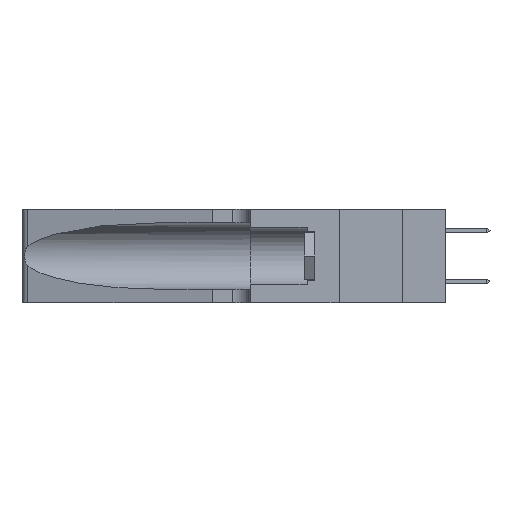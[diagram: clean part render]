
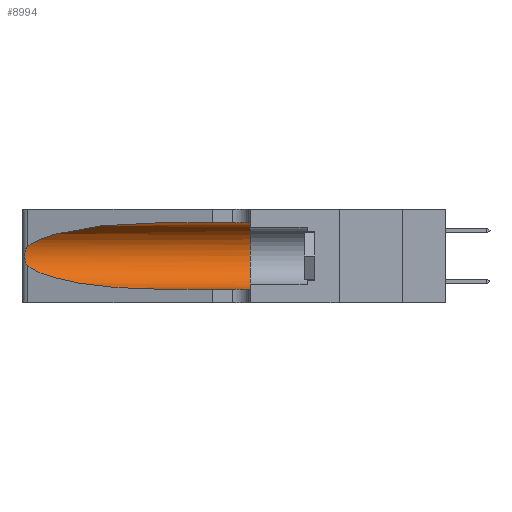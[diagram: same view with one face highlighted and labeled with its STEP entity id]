
A CAD part, left-side view. The second image highlights one B-rep face of the part: STEP entity #8994.
In plain terms, the highlighted cylindrical face has radius 3.308 mm (diameter 6.617 mm), a partial arc.
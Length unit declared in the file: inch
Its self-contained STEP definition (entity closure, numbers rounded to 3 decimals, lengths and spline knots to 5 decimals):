
#883 = ORIENTED_EDGE ( 'NONE', *, *, #2838, .T. ) ;
#949 = CARTESIAN_POINT ( 'NONE',  ( 0.18966, 0.96281, 0.05475 ) ) ;
#1196 = CARTESIAN_POINT ( 'NONE',  ( 0.1305, 0.72297, 0.31525 ) ) ;
#1258 = CARTESIAN_POINT ( 'NONE',  ( 0.2373, 1.15595, 0.28018 ) ) ;
#1338 = LINE ( 'NONE', #2550, #20241 ) ;
#1726 = LINE ( 'NONE', #13291, #14438 ) ;
#1808 = CARTESIAN_POINT ( 'NONE',  ( 0.25789, 1.23486, 0.15765 ) ) ;
#2550 = CARTESIAN_POINT ( 'NONE',  ( 0.1305, 1.61858, 0.05475 ) ) ;
#2621 = CARTESIAN_POINT ( 'NONE',  ( 0.1305, 0.72297, 0.05475 ) ) ;
#2838 = EDGE_CURVE ( 'NONE', #6435, #15644, #19381, .T. ) ;
#2980 = ORIENTED_EDGE ( 'NONE', *, *, #15536, .T. ) ;
#3025 = DIRECTION ( 'NONE',  ( 0., -1., 0. ) ) ;
#3553 = CARTESIAN_POINT ( 'NONE',  ( 0.1305, 1.61858, 0.185 ) ) ;
#4504 = CARTESIAN_POINT ( 'NONE',  ( 0.25487, 1.22718, 0.14631 ) ) ;
#5273 = CARTESIAN_POINT ( 'NONE',  ( 0.25639, 1.23184, 0.21858 ) ) ;
#5426 = DIRECTION ( 'NONE',  ( 0., -1., 0. ) ) ;
#5427 = CARTESIAN_POINT ( 'NONE',  ( 0.1305, 0.35, 0.31525 ) ) ;
#5573 = CARTESIAN_POINT ( 'NONE',  ( 0.1305, 0.35, 0.05475 ) ) ;
#5808 = CARTESIAN_POINT ( 'NONE',  ( 0.25487, 1.22718, 0.22369 ) ) ;
#6435 = VERTEX_POINT ( 'NONE', #1196 ) ;
#6538 = CARTESIAN_POINT ( 'NONE',  ( 0.18966, 0.96281, 0.31525 ) ) ;
#6994 = CARTESIAN_POINT ( 'NONE',  ( 0.25487, 1.22718, 0.14631 ) ) ;
#7041 =( BOUNDED_CURVE ( )  B_SPLINE_CURVE ( 3, ( #4504, #11273, #949, #2621 ),
 .UNSPECIFIED., .F., .T. ) 
 B_SPLINE_CURVE_WITH_KNOTS ( ( 4, 4 ),
 ( 3.44316, 4.71239 ),
 .UNSPECIFIED. ) 
 CURVE ( )  GEOMETRIC_REPRESENTATION_ITEM ( )  RATIONAL_B_SPLINE_CURVE ( ( 1., 0.87, 0.87, 1. ) ) 
 REPRESENTATION_ITEM ( '' )  );
#7078 = CARTESIAN_POINT ( 'NONE',  ( 0.25555, 1.22993, 0.14849 ) ) ;
#7148 = CARTESIAN_POINT ( 'NONE',  ( 0.26075, 1.23896, 0.178 ) ) ;
#8267 = CARTESIAN_POINT ( 'NONE',  ( 0.25487, 1.22718, 0.22369 ) ) ;
#8703 = DIRECTION ( 'NONE',  ( 0., 1., 0. ) ) ;
#8822 = CARTESIAN_POINT ( 'NONE',  ( 0.25854, 1.2359, 0.20912 ) ) ;
#8981 = CARTESIAN_POINT ( 'NONE',  ( 0.26018, 1.23835, 0.19895 ) ) ;
#8994 = ADVANCED_FACE ( 'NONE', ( #20002 ), #15130, .F. ) ;
#9029 = CIRCLE ( 'NONE', #16340, 0.13025 ) ;
#9143 = ORIENTED_EDGE ( 'NONE', *, *, #13615, .T. ) ;
#9603 = EDGE_LOOP ( 'NONE', ( #883, #2980, #13692, #9143, #16272, #11738 ) ) ;
#10315 = EDGE_CURVE ( 'NONE', #12805, #20885, #9029, .T. ) ;
#10669 = EDGE_CURVE ( 'NONE', #6435, #12805, #1726, .T. ) ;
#11104 = AXIS2_PLACEMENT_3D ( 'NONE', #3553, #5426, #17498 ) ;
#11273 = CARTESIAN_POINT ( 'NONE',  ( 0.2373, 1.15595, 0.08982 ) ) ;
#11354 = CARTESIAN_POINT ( 'NONE',  ( 0.25487, 1.22718, 0.14631 ) ) ;
#11588 = CARTESIAN_POINT ( 'NONE',  ( 0.1305, 0.72297, 0.31525 ) ) ;
#11738 = ORIENTED_EDGE ( 'NONE', *, *, #10669, .F. ) ;
#11903 = CARTESIAN_POINT ( 'NONE',  ( 0.25555, 1.22994, 0.2215 ) ) ;
#12063 = CARTESIAN_POINT ( 'NONE',  ( 0.25487, 1.22718, 0.22369 ) ) ;
#12453 = CARTESIAN_POINT ( 'NONE',  ( 0.25856, 1.23593, 0.16098 ) ) ;
#12805 = VERTEX_POINT ( 'NONE', #5427 ) ;
#13291 = CARTESIAN_POINT ( 'NONE',  ( 0.1305, 1.61858, 0.31525 ) ) ;
#13615 = EDGE_CURVE ( 'NONE', #21228, #20885, #1338, .T. ) ;
#13692 = ORIENTED_EDGE ( 'NONE', *, *, #13705, .T. ) ;
#13705 = EDGE_CURVE ( 'NONE', #20971, #21228, #7041, .T. ) ;
#14438 = VECTOR ( 'NONE', #3025, 39.37008 ) ;
#15130 = CYLINDRICAL_SURFACE ( 'NONE', #11104, 0.13025 ) ;
#15491 = DIRECTION ( 'NONE',  ( 0., 0., 1. ) ) ;
#15536 = EDGE_CURVE ( 'NONE', #15644, #20971, #17414, .T. ) ;
#15644 = VERTEX_POINT ( 'NONE', #5808 ) ;
#15763 = CARTESIAN_POINT ( 'NONE',  ( 0.25787, 1.23484, 0.2124 ) ) ;
#16056 = DIRECTION ( 'NONE',  ( 0., -1., 0. ) ) ;
#16272 = ORIENTED_EDGE ( 'NONE', *, *, #10315, .F. ) ;
#16340 = AXIS2_PLACEMENT_3D ( 'NONE', #17210, #8703, #15491 ) ;
#17210 = CARTESIAN_POINT ( 'NONE',  ( 0.1305, 0.35, 0.185 ) ) ;
#17336 = CARTESIAN_POINT ( 'NONE',  ( 0.26017, 1.23833, 0.17102 ) ) ;
#17414 = B_SPLINE_CURVE_WITH_KNOTS ( 'NONE', 3,
 ( #12063, #11903, #5273, #15763, #8822, #8981, #19312, #7148, #17336, #12453, #1808, #17413, #7078, #6994 ),
 .UNSPECIFIED., .F., .F.,
 ( 4, 2, 2, 2, 2, 2, 4 ),
 ( 0., 0.00027, 0.00053, 0.00107, 0.0016, 0.00187, 0.00214 ),
 .UNSPECIFIED. ) ;
#17413 = CARTESIAN_POINT ( 'NONE',  ( 0.25639, 1.23186, 0.15144 ) ) ;
#17498 = DIRECTION ( 'NONE',  ( 0., 0., -1. ) ) ;
#18822 = CARTESIAN_POINT ( 'NONE',  ( 0.1305, 0.72297, 0.05475 ) ) ;
#19312 = CARTESIAN_POINT ( 'NONE',  ( 0.26075, 1.23896, 0.19203 ) ) ;
#19381 =( BOUNDED_CURVE ( )  B_SPLINE_CURVE ( 3, ( #11588, #6538, #1258, #8267 ),
 .UNSPECIFIED., .F., .F. ) 
 B_SPLINE_CURVE_WITH_KNOTS ( ( 4, 4 ),
 ( 1.5708, 2.84003 ),
 .UNSPECIFIED. ) 
 CURVE ( )  GEOMETRIC_REPRESENTATION_ITEM ( )  RATIONAL_B_SPLINE_CURVE ( ( 1., 0.87, 0.87, 1. ) ) 
 REPRESENTATION_ITEM ( '' )  );
#20002 = FACE_OUTER_BOUND ( 'NONE', #9603, .T. ) ;
#20241 = VECTOR ( 'NONE', #16056, 39.37008 ) ;
#20885 = VERTEX_POINT ( 'NONE', #5573 ) ;
#20971 = VERTEX_POINT ( 'NONE', #11354 ) ;
#21228 = VERTEX_POINT ( 'NONE', #18822 ) ;
